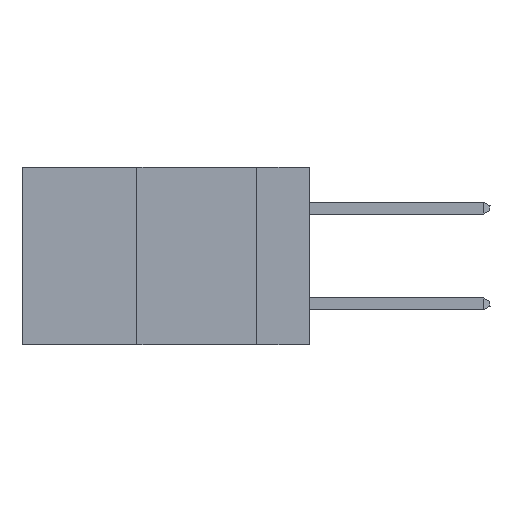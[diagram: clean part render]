
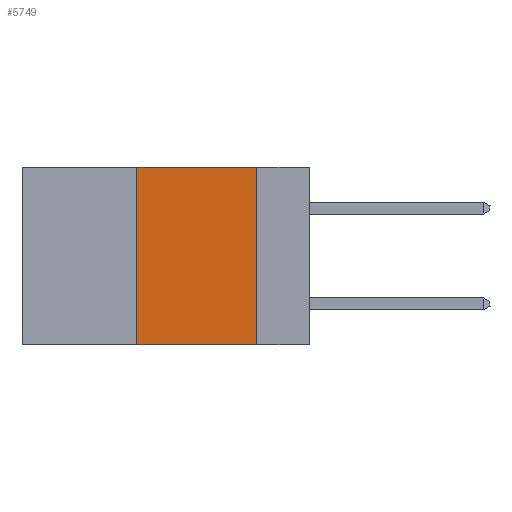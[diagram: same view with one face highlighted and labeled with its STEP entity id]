
A CAD part, left-side view. The second image highlights one B-rep face of the part: STEP entity #5749.
In plain terms, the highlighted planar face has unit normal (-1, 0, 0).
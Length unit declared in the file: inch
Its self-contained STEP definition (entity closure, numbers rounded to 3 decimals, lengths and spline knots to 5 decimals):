
#2181 = VERTEX_POINT ( 'NONE', #15607 ) ;
#2832 = EDGE_CURVE ( 'NONE', #16205, #2181, #11571, .T. ) ;
#4277 = EDGE_LOOP ( 'NONE', ( #14000, #17429, #16880, #6988 ) ) ;
#4838 = LINE ( 'NONE', #15155, #11211 ) ;
#5168 = DIRECTION ( 'NONE',  ( 0., 0., -1. ) ) ;
#5227 = PLANE ( 'NONE',  #14748 ) ;
#5330 = VERTEX_POINT ( 'NONE', #9620 ) ;
#5472 = CARTESIAN_POINT ( 'NONE',  ( 0., 0.11, 0. ) ) ;
#5749 = ADVANCED_FACE ( 'NONE', ( #17590 ), #5227, .F. ) ;
#6939 = EDGE_CURVE ( 'NONE', #2181, #5330, #14368, .T. ) ;
#6988 = ORIENTED_EDGE ( 'NONE', *, *, #15730, .T. ) ;
#8011 = LINE ( 'NONE', #9524, #10962 ) ;
#8090 = CARTESIAN_POINT ( 'NONE',  ( 0., 0.36, 0. ) ) ;
#8154 = DIRECTION ( 'NONE',  ( 0., 0., 1. ) ) ;
#8164 = CARTESIAN_POINT ( 'NONE',  ( 0., 0.36, -0.37 ) ) ;
#9455 = DIRECTION ( 'NONE',  ( 1., 0., 0. ) ) ;
#9524 = CARTESIAN_POINT ( 'NONE',  ( 0., 0.36, 0. ) ) ;
#9620 = CARTESIAN_POINT ( 'NONE',  ( 0., 0.11, -0.37 ) ) ;
#10838 = DIRECTION ( 'NONE',  ( 0., -1., 0. ) ) ;
#10962 = VECTOR ( 'NONE', #8154, 39.37008 ) ;
#11211 = VECTOR ( 'NONE', #10838, 39.37008 ) ;
#11571 = LINE ( 'NONE', #17416, #14968 ) ;
#12921 = DIRECTION ( 'NONE',  ( 0., 0., -1. ) ) ;
#12990 = DIRECTION ( 'NONE',  ( 0., -1., 0. ) ) ;
#14000 = ORIENTED_EDGE ( 'NONE', *, *, #6939, .F. ) ;
#14368 = LINE ( 'NONE', #5472, #16381 ) ;
#14748 = AXIS2_PLACEMENT_3D ( 'NONE', #15376, #9455, #5168 ) ;
#14968 = VECTOR ( 'NONE', #12990, 39.37008 ) ;
#15155 = CARTESIAN_POINT ( 'NONE',  ( 0., 0.6, -0.37 ) ) ;
#15266 = VERTEX_POINT ( 'NONE', #8164 ) ;
#15376 = CARTESIAN_POINT ( 'NONE',  ( 0., 0.6, 0. ) ) ;
#15607 = CARTESIAN_POINT ( 'NONE',  ( 0., 0.11, 0. ) ) ;
#15730 = EDGE_CURVE ( 'NONE', #15266, #5330, #4838, .T. ) ;
#16204 = EDGE_CURVE ( 'NONE', #15266, #16205, #8011, .T. ) ;
#16205 = VERTEX_POINT ( 'NONE', #8090 ) ;
#16381 = VECTOR ( 'NONE', #12921, 39.37008 ) ;
#16880 = ORIENTED_EDGE ( 'NONE', *, *, #16204, .F. ) ;
#17416 = CARTESIAN_POINT ( 'NONE',  ( 0., 0.6, 0. ) ) ;
#17429 = ORIENTED_EDGE ( 'NONE', *, *, #2832, .F. ) ;
#17590 = FACE_OUTER_BOUND ( 'NONE', #4277, .T. ) ;
